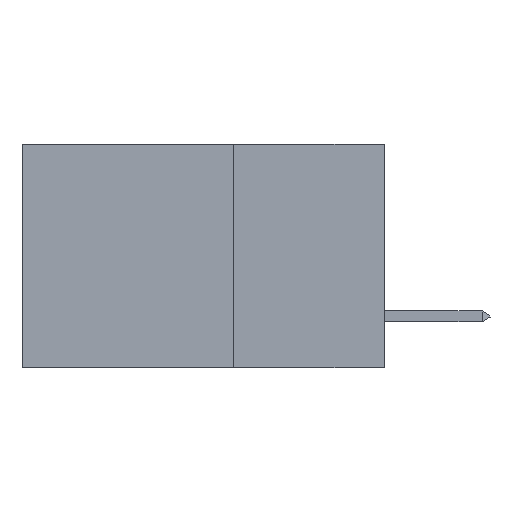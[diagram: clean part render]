
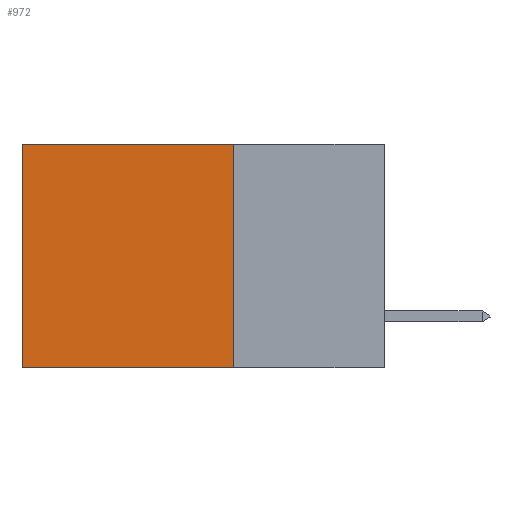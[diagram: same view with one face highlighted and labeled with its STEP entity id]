
A CAD part, left-side view. The second image highlights one B-rep face of the part: STEP entity #972.
In plain terms, the highlighted planar face has unit normal (-1, 0, 0).
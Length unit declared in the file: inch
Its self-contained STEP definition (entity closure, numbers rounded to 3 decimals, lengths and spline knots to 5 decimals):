
#253 = EDGE_CURVE ( 'NONE', #3147, #6197, #385, .T. ) ;
#385 = LINE ( 'NONE', #7132, #7951 ) ;
#388 = FACE_OUTER_BOUND ( 'NONE', #10138, .T. ) ;
#903 = CARTESIAN_POINT ( 'NONE',  ( 0.2875, 0.6, -0.37 ) ) ;
#972 = ADVANCED_FACE ( 'NONE', ( #388 ), #10263, .F. ) ;
#1013 = DIRECTION ( 'NONE',  ( 0., 0., -1. ) ) ;
#1116 = DIRECTION ( 'NONE',  ( 0., 0., -1. ) ) ;
#1746 = LINE ( 'NONE', #9541, #5236 ) ;
#3147 = VERTEX_POINT ( 'NONE', #14318 ) ;
#4941 = CARTESIAN_POINT ( 'NONE',  ( 0.2875, 0.25, 0. ) ) ;
#5236 = VECTOR ( 'NONE', #6583, 39.37008 ) ;
#6197 = VERTEX_POINT ( 'NONE', #903 ) ;
#6570 = AXIS2_PLACEMENT_3D ( 'NONE', #10501, #10175, #10108 ) ;
#6583 = DIRECTION ( 'NONE',  ( 0., 1., 0. ) ) ;
#7132 = CARTESIAN_POINT ( 'NONE',  ( 0.2875, 0.6, 0. ) ) ;
#7951 = VECTOR ( 'NONE', #1013, 39.37008 ) ;
#8134 = CARTESIAN_POINT ( 'NONE',  ( 0.2875, 0.25, 0. ) ) ;
#8458 = ORIENTED_EDGE ( 'NONE', *, *, #253, .T. ) ;
#8599 = VECTOR ( 'NONE', #17143, 39.37008 ) ;
#8829 = EDGE_CURVE ( 'NONE', #12068, #3147, #16526, .T. ) ;
#9010 = ORIENTED_EDGE ( 'NONE', *, *, #8829, .T. ) ;
#9211 = ORIENTED_EDGE ( 'NONE', *, *, #16430, .F. ) ;
#9449 = EDGE_CURVE ( 'NONE', #17687, #6197, #1746, .T. ) ;
#9541 = CARTESIAN_POINT ( 'NONE',  ( 0.2875, 0.25, -0.37 ) ) ;
#10105 = CARTESIAN_POINT ( 'NONE',  ( 0.2875, 0.25, 0. ) ) ;
#10108 = DIRECTION ( 'NONE',  ( 0., 0., -1. ) ) ;
#10138 = EDGE_LOOP ( 'NONE', ( #8458, #12796, #9211, #9010 ) ) ;
#10175 = DIRECTION ( 'NONE',  ( 1., 0., 0. ) ) ;
#10263 = PLANE ( 'NONE',  #6570 ) ;
#10501 = CARTESIAN_POINT ( 'NONE',  ( 0.2875, 0.25, 0. ) ) ;
#11153 = LINE ( 'NONE', #10105, #12116 ) ;
#12068 = VERTEX_POINT ( 'NONE', #4941 ) ;
#12116 = VECTOR ( 'NONE', #1116, 39.37008 ) ;
#12796 = ORIENTED_EDGE ( 'NONE', *, *, #9449, .F. ) ;
#14056 = CARTESIAN_POINT ( 'NONE',  ( 0.2875, 0.25, -0.37 ) ) ;
#14318 = CARTESIAN_POINT ( 'NONE',  ( 0.2875, 0.6, 0. ) ) ;
#16430 = EDGE_CURVE ( 'NONE', #12068, #17687, #11153, .T. ) ;
#16526 = LINE ( 'NONE', #8134, #8599 ) ;
#17143 = DIRECTION ( 'NONE',  ( 0., 1., 0. ) ) ;
#17687 = VERTEX_POINT ( 'NONE', #14056 ) ;
